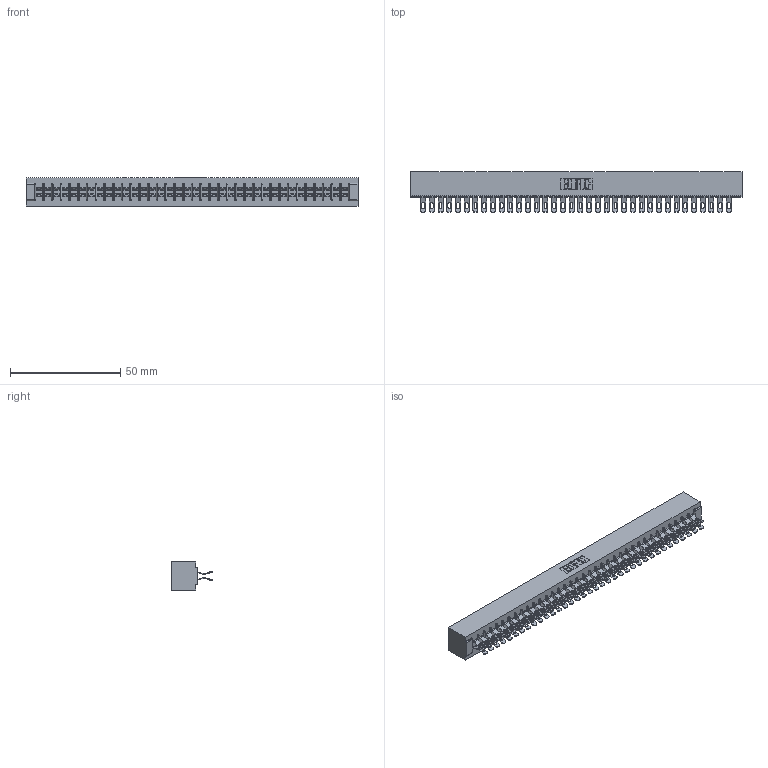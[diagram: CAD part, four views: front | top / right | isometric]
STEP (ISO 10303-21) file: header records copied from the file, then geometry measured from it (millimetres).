
FILE_DESCRIPTION (( 'STEP AP203' ), '1' );
FILE_NAME ('305-072-555-501.STEP', '2019-09-10T06:23:05', ( '' ), ( '' ), 'SwSTEP 2.0', 'SolidWorks 2016', '' );
FILE_SCHEMA (( 'CONFIG_CONTROL_DESIGN' ));
Length unit declared in the file: inch
Products named in the file (3): 305-072-555-501; 305 Part_No Mounting; 305-290-001_555
Assembly tree (73 placements, depth 2):
  305-072-555-501
    305 Part_No Mounting
    305-290-001_555  x72
Bounding box: 150.52 x 18.41 x 12.7 mm (x, y, z)
Volume: 15866.3 mm3; surface area: 22607.6 mm2
Topology: 73 solids, 73 shells, 4860 faces, 14512 edges, 9480 vertices
Faces by surface type: plane 2368, cylinder 2348, sphere 144
Entity records: 40055 total; most frequent: CARTESIAN_POINT 6644, ORIENTED_EDGE 6584, DIRECTION 6424, EDGE_CURVE 3292, LINE 2640, VECTOR 2640, VERTEX_POINT 2096, AXIS2_PLACEMENT_3D 1892
